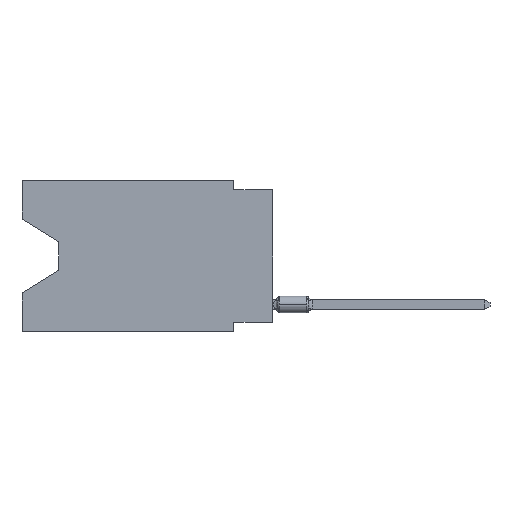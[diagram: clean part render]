
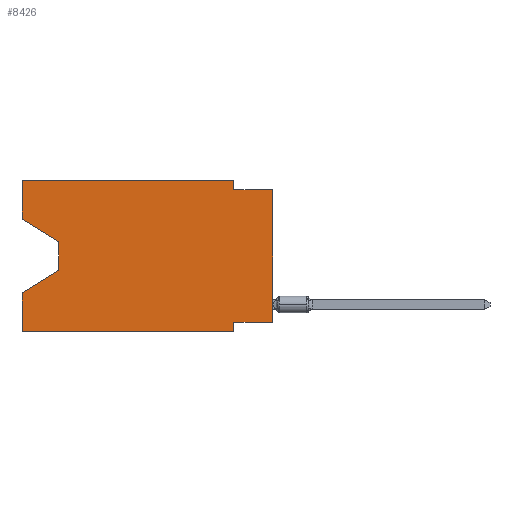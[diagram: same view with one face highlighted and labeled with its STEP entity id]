
A CAD part, left-side view. The second image highlights one B-rep face of the part: STEP entity #8426.
In plain terms, the highlighted planar face has unit normal (-1, 0, 0).
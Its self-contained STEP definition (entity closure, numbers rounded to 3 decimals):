
#97 = DIRECTION ( 'NONE',  ( 0., 0., -1. ) ) ;
#105 = EDGE_CURVE ( 'NONE', #13868, #8978, #5120, .T. ) ;
#557 = CARTESIAN_POINT ( 'NONE',  ( 0., 13.97, -5.893 ) ) ;
#694 = EDGE_CURVE ( 'NONE', #1707, #2205, #8226, .T. ) ;
#759 = EDGE_CURVE ( 'NONE', #8978, #8773, #10900, .T. ) ;
#869 = CARTESIAN_POINT ( 'NONE',  ( 0., 0., -9.271 ) ) ;
#1190 = CARTESIAN_POINT ( 'NONE',  ( 0., 16.383, 0. ) ) ;
#1208 = VECTOR ( 'NONE', #12861, 1000. ) ;
#1334 = DIRECTION ( 'NONE',  ( 0., 0., -1. ) ) ;
#1501 = ORIENTED_EDGE ( 'NONE', *, *, #759, .F. ) ;
#1510 = VECTOR ( 'NONE', #7205, 1000. ) ;
#1525 = VECTOR ( 'NONE', #3254, 1000. ) ;
#1707 = VERTEX_POINT ( 'NONE', #2982 ) ;
#1866 = DIRECTION ( 'NONE',  ( 0., -0.855, -0.519 ) ) ;
#1958 = ORIENTED_EDGE ( 'NONE', *, *, #105, .F. ) ;
#2205 = VERTEX_POINT ( 'NONE', #8511 ) ;
#2405 = EDGE_CURVE ( 'NONE', #14899, #7296, #5003, .T. ) ;
#2407 = CARTESIAN_POINT ( 'NONE',  ( 0., 16.383, -9.906 ) ) ;
#2502 = DIRECTION ( 'NONE',  ( 0., -1., 0. ) ) ;
#2534 = LINE ( 'NONE', #10933, #3424 ) ;
#2589 = EDGE_LOOP ( 'NONE', ( #10514, #12669, #9085, #7782, #9369, #11376, #8420, #7452, #6224, #1501, #1958, #7272 ) ) ;
#2620 = VERTEX_POINT ( 'NONE', #11723 ) ;
#2755 = VERTEX_POINT ( 'NONE', #2960 ) ;
#2960 = CARTESIAN_POINT ( 'NONE',  ( 0., 0., -0.635 ) ) ;
#2982 = CARTESIAN_POINT ( 'NONE',  ( 0., 2.54, -9.271 ) ) ;
#3134 = VECTOR ( 'NONE', #10824, 1000. ) ;
#3168 = DIRECTION ( 'NONE',  ( 0., -1., 0. ) ) ;
#3254 = DIRECTION ( 'NONE',  ( 0., 0., 1. ) ) ;
#3424 = VECTOR ( 'NONE', #9765, 1000. ) ;
#3864 = LINE ( 'NONE', #4890, #9211 ) ;
#3968 = EDGE_CURVE ( 'NONE', #2620, #10113, #3864, .T. ) ;
#4237 = CARTESIAN_POINT ( 'NONE',  ( 0., 0., 0. ) ) ;
#4307 = LINE ( 'NONE', #9229, #14081 ) ;
#4465 = LINE ( 'NONE', #2407, #1510 ) ;
#4532 = VERTEX_POINT ( 'NONE', #5606 ) ;
#4890 = CARTESIAN_POINT ( 'NONE',  ( 0., 13.97, -4.013 ) ) ;
#5003 = LINE ( 'NONE', #7424, #9874 ) ;
#5049 = CARTESIAN_POINT ( 'NONE',  ( 0., 16.383, -9.906 ) ) ;
#5118 = CARTESIAN_POINT ( 'NONE',  ( 0., 2.54, 0. ) ) ;
#5120 = LINE ( 'NONE', #9733, #14680 ) ;
#5318 = DIRECTION ( 'NONE',  ( 0., 0., 1. ) ) ;
#5579 = CARTESIAN_POINT ( 'NONE',  ( 0., 16.383, 0. ) ) ;
#5606 = CARTESIAN_POINT ( 'NONE',  ( 0., 16.383, -2.546 ) ) ;
#6116 = VECTOR ( 'NONE', #3168, 1000. ) ;
#6217 = VECTOR ( 'NONE', #10453, 1000. ) ;
#6224 = ORIENTED_EDGE ( 'NONE', *, *, #7091, .F. ) ;
#6240 = DIRECTION ( 'NONE',  ( 1., 0., 0. ) ) ;
#7091 = EDGE_CURVE ( 'NONE', #8773, #2755, #12528, .T. ) ;
#7168 = CARTESIAN_POINT ( 'NONE',  ( 0., 16.383, -7.36 ) ) ;
#7205 = DIRECTION ( 'NONE',  ( 0., -1., 0. ) ) ;
#7272 = ORIENTED_EDGE ( 'NONE', *, *, #9473, .F. ) ;
#7296 = VERTEX_POINT ( 'NONE', #7168 ) ;
#7424 = CARTESIAN_POINT ( 'NONE',  ( 0., 16.383, 0. ) ) ;
#7452 = ORIENTED_EDGE ( 'NONE', *, *, #10642, .T. ) ;
#7782 = ORIENTED_EDGE ( 'NONE', *, *, #2405, .F. ) ;
#7873 = LINE ( 'NONE', #869, #6217 ) ;
#8226 = LINE ( 'NONE', #9488, #9391 ) ;
#8420 = ORIENTED_EDGE ( 'NONE', *, *, #8724, .F. ) ;
#8426 = ADVANCED_FACE ( 'NONE', ( #13056 ), #13215, .F. ) ;
#8443 = EDGE_CURVE ( 'NONE', #10113, #7296, #2534, .T. ) ;
#8511 = CARTESIAN_POINT ( 'NONE',  ( 0., 2.54, -9.906 ) ) ;
#8724 = EDGE_CURVE ( 'NONE', #9166, #1707, #7873, .T. ) ;
#8773 = VERTEX_POINT ( 'NONE', #10681 ) ;
#8978 = VERTEX_POINT ( 'NONE', #14871 ) ;
#9085 = ORIENTED_EDGE ( 'NONE', *, *, #8443, .T. ) ;
#9166 = VERTEX_POINT ( 'NONE', #11842 ) ;
#9211 = VECTOR ( 'NONE', #1334, 1000. ) ;
#9229 = CARTESIAN_POINT ( 'NONE',  ( 0., 16.383, -2.546 ) ) ;
#9315 = LINE ( 'NONE', #4237, #1208 ) ;
#9369 = ORIENTED_EDGE ( 'NONE', *, *, #12790, .T. ) ;
#9391 = VECTOR ( 'NONE', #12949, 1000. ) ;
#9473 = EDGE_CURVE ( 'NONE', #4532, #13868, #10554, .T. ) ;
#9488 = CARTESIAN_POINT ( 'NONE',  ( 0., 2.54, -9.906 ) ) ;
#9733 = CARTESIAN_POINT ( 'NONE',  ( 0., 16.383, 0. ) ) ;
#9765 = DIRECTION ( 'NONE',  ( 0., 0.855, -0.519 ) ) ;
#9874 = VECTOR ( 'NONE', #5318, 1000. ) ;
#10113 = VERTEX_POINT ( 'NONE', #557 ) ;
#10453 = DIRECTION ( 'NONE',  ( 0., 1., 0. ) ) ;
#10514 = ORIENTED_EDGE ( 'NONE', *, *, #14043, .T. ) ;
#10554 = LINE ( 'NONE', #14106, #1525 ) ;
#10642 = EDGE_CURVE ( 'NONE', #9166, #2755, #9315, .T. ) ;
#10681 = CARTESIAN_POINT ( 'NONE',  ( 0., 2.54, -0.635 ) ) ;
#10824 = DIRECTION ( 'NONE',  ( 0., 0., -1. ) ) ;
#10900 = LINE ( 'NONE', #5118, #3134 ) ;
#10933 = CARTESIAN_POINT ( 'NONE',  ( 0., 13.97, -5.893 ) ) ;
#10962 = AXIS2_PLACEMENT_3D ( 'NONE', #1190, #6240, #97 ) ;
#11376 = ORIENTED_EDGE ( 'NONE', *, *, #694, .F. ) ;
#11723 = CARTESIAN_POINT ( 'NONE',  ( 0., 13.97, -4.013 ) ) ;
#11842 = CARTESIAN_POINT ( 'NONE',  ( 0., 0., -9.271 ) ) ;
#12528 = LINE ( 'NONE', #14826, #6116 ) ;
#12669 = ORIENTED_EDGE ( 'NONE', *, *, #3968, .T. ) ;
#12790 = EDGE_CURVE ( 'NONE', #14899, #2205, #4465, .T. ) ;
#12861 = DIRECTION ( 'NONE',  ( 0., 0., 1. ) ) ;
#12949 = DIRECTION ( 'NONE',  ( 0., 0., -1. ) ) ;
#13056 = FACE_OUTER_BOUND ( 'NONE', #2589, .T. ) ;
#13215 = PLANE ( 'NONE',  #10962 ) ;
#13868 = VERTEX_POINT ( 'NONE', #5579 ) ;
#14043 = EDGE_CURVE ( 'NONE', #4532, #2620, #4307, .T. ) ;
#14081 = VECTOR ( 'NONE', #1866, 1000. ) ;
#14106 = CARTESIAN_POINT ( 'NONE',  ( 0., 16.383, 0. ) ) ;
#14680 = VECTOR ( 'NONE', #2502, 1000. ) ;
#14826 = CARTESIAN_POINT ( 'NONE',  ( 0., 0., -0.635 ) ) ;
#14871 = CARTESIAN_POINT ( 'NONE',  ( 0., 2.54, 0. ) ) ;
#14899 = VERTEX_POINT ( 'NONE', #5049 ) ;
